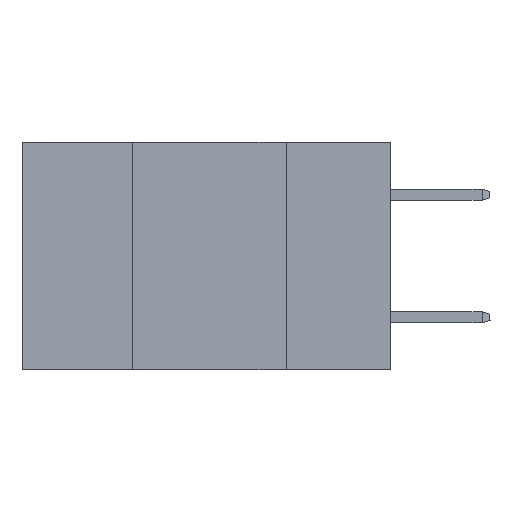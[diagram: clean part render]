
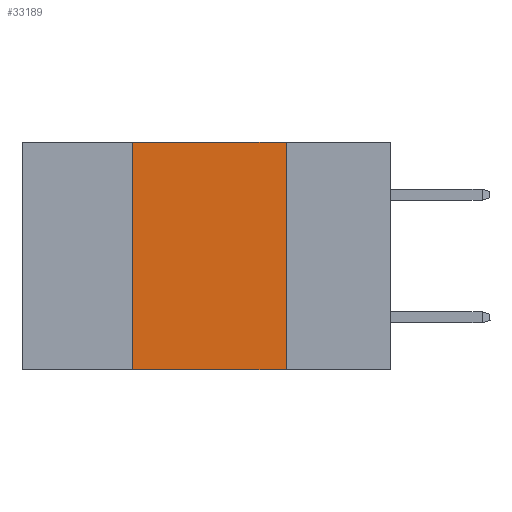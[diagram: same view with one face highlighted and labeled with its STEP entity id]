
A CAD part, left-side view. The second image highlights one B-rep face of the part: STEP entity #33189.
In plain terms, the highlighted planar face has unit normal (-1, 0, 0).
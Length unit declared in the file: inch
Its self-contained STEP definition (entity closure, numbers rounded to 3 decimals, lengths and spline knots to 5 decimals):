
#375 = EDGE_CURVE ( 'NONE', #44045, #25414, #7511, .T. ) ;
#981 = DIRECTION ( 'NONE',  ( 1., 0., 0. ) ) ;
#1717 = ORIENTED_EDGE ( 'NONE', *, *, #2756, .F. ) ;
#2756 = EDGE_CURVE ( 'NONE', #13097, #25414, #38202, .T. ) ;
#4263 = CARTESIAN_POINT ( 'NONE',  ( 0., 0.17, 0. ) ) ;
#7511 = LINE ( 'NONE', #29275, #46475 ) ;
#8739 = ORIENTED_EDGE ( 'NONE', *, *, #44498, .F. ) ;
#8747 = VECTOR ( 'NONE', #16495, 39.37008 ) ;
#8783 = ORIENTED_EDGE ( 'NONE', *, *, #18562, .F. ) ;
#9196 = DIRECTION ( 'NONE',  ( 0., 0., -1. ) ) ;
#10336 = CARTESIAN_POINT ( 'NONE',  ( 0., 0.17, 0. ) ) ;
#10421 = CARTESIAN_POINT ( 'NONE',  ( 0., 0.42, 0. ) ) ;
#11509 = AXIS2_PLACEMENT_3D ( 'NONE', #44626, #981, #33887 ) ;
#12735 = CARTESIAN_POINT ( 'NONE',  ( 0., 0.6, 0. ) ) ;
#13047 = DIRECTION ( 'NONE',  ( 0., -1., 0. ) ) ;
#13097 = VERTEX_POINT ( 'NONE', #10336 ) ;
#16495 = DIRECTION ( 'NONE',  ( 0., 0., 1. ) ) ;
#18562 = EDGE_CURVE ( 'NONE', #36224, #13097, #23031, .T. ) ;
#19434 = CARTESIAN_POINT ( 'NONE',  ( 0., 0.42, -0.37 ) ) ;
#23031 = LINE ( 'NONE', #12735, #35050 ) ;
#25414 = VERTEX_POINT ( 'NONE', #39250 ) ;
#26327 = CARTESIAN_POINT ( 'NONE',  ( 0., 0.42, 0. ) ) ;
#27796 = EDGE_LOOP ( 'NONE', ( #1717, #8783, #8739, #32141 ) ) ;
#29275 = CARTESIAN_POINT ( 'NONE',  ( 0., 0.6, -0.37 ) ) ;
#29948 = LINE ( 'NONE', #26327, #8747 ) ;
#31529 = FACE_OUTER_BOUND ( 'NONE', #27796, .T. ) ;
#32141 = ORIENTED_EDGE ( 'NONE', *, *, #375, .T. ) ;
#33189 = ADVANCED_FACE ( 'NONE', ( #31529 ), #41730, .F. ) ;
#33549 = DIRECTION ( 'NONE',  ( 0., -1., 0. ) ) ;
#33887 = DIRECTION ( 'NONE',  ( 0., 0., -1. ) ) ;
#35050 = VECTOR ( 'NONE', #13047, 39.37008 ) ;
#36224 = VERTEX_POINT ( 'NONE', #10421 ) ;
#38202 = LINE ( 'NONE', #4263, #39343 ) ;
#39250 = CARTESIAN_POINT ( 'NONE',  ( 0., 0.17, -0.37 ) ) ;
#39343 = VECTOR ( 'NONE', #9196, 39.37008 ) ;
#41730 = PLANE ( 'NONE',  #11509 ) ;
#44045 = VERTEX_POINT ( 'NONE', #19434 ) ;
#44498 = EDGE_CURVE ( 'NONE', #44045, #36224, #29948, .T. ) ;
#44626 = CARTESIAN_POINT ( 'NONE',  ( 0., 0.6, 0. ) ) ;
#46475 = VECTOR ( 'NONE', #33549, 39.37008 ) ;
